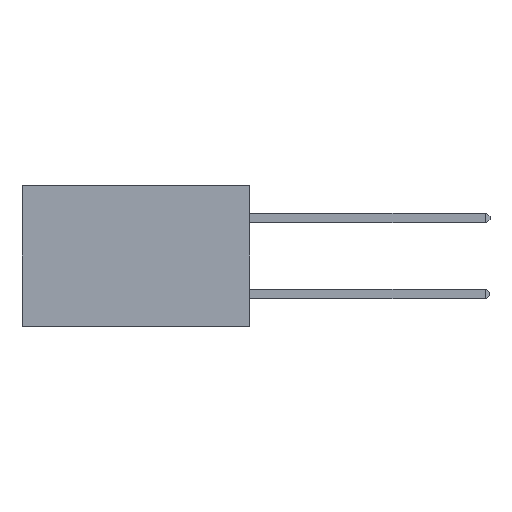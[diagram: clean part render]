
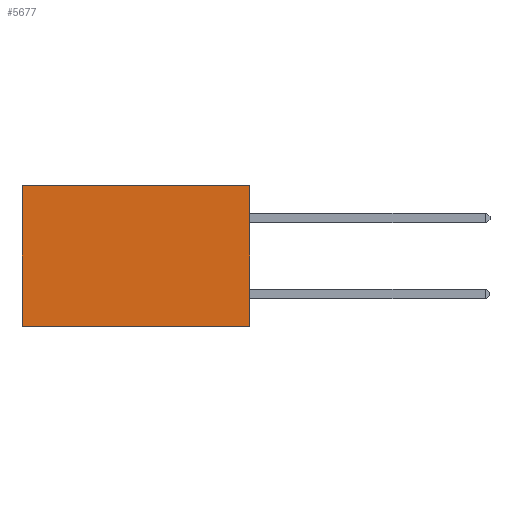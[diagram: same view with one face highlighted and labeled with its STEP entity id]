
A CAD part, left-side view. The second image highlights one B-rep face of the part: STEP entity #5677.
In plain terms, the highlighted planar face has unit normal (-1, 0, 0).
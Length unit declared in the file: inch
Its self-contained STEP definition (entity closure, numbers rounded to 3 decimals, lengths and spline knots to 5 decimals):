
#336 = CARTESIAN_POINT ( 'NONE',  ( 0.2875, 0.6, 0. ) ) ;
#605 = CARTESIAN_POINT ( 'NONE',  ( 0.2875, 0.6, 0. ) ) ;
#1169 = ORIENTED_EDGE ( 'NONE', *, *, #3508, .T. ) ;
#1212 = VECTOR ( 'NONE', #2059, 39.37008 ) ;
#2059 = DIRECTION ( 'NONE',  ( 0., 0., -1. ) ) ;
#2659 = FACE_OUTER_BOUND ( 'NONE', #3491, .T. ) ;
#2679 = CARTESIAN_POINT ( 'NONE',  ( 0.2875, 0., 0. ) ) ;
#2839 = ORIENTED_EDGE ( 'NONE', *, *, #12120, .T. ) ;
#3178 = EDGE_CURVE ( 'NONE', #4184, #4004, #9145, .T. ) ;
#3382 = DIRECTION ( 'NONE',  ( 0., 1., 0. ) ) ;
#3413 = CARTESIAN_POINT ( 'NONE',  ( 0.2875, 0., -0.37 ) ) ;
#3491 = EDGE_LOOP ( 'NONE', ( #2839, #12076, #4871, #1169 ) ) ;
#3508 = EDGE_CURVE ( 'NONE', #4184, #9931, #11908, .T. ) ;
#3695 = LINE ( 'NONE', #336, #11287 ) ;
#3715 = AXIS2_PLACEMENT_3D ( 'NONE', #2679, #11547, #5685 ) ;
#4004 = VERTEX_POINT ( 'NONE', #6241 ) ;
#4053 = VECTOR ( 'NONE', #10261, 39.37008 ) ;
#4184 = VERTEX_POINT ( 'NONE', #4662 ) ;
#4239 = EDGE_CURVE ( 'NONE', #4004, #8401, #5621, .T. ) ;
#4662 = CARTESIAN_POINT ( 'NONE',  ( 0.2875, 0., 0. ) ) ;
#4871 = ORIENTED_EDGE ( 'NONE', *, *, #3178, .F. ) ;
#5621 = LINE ( 'NONE', #3413, #8037 ) ;
#5677 = ADVANCED_FACE ( 'NONE', ( #2659 ), #6687, .F. ) ;
#5685 = DIRECTION ( 'NONE',  ( 0., 0., -1. ) ) ;
#6241 = CARTESIAN_POINT ( 'NONE',  ( 0.2875, 0., -0.37 ) ) ;
#6687 = PLANE ( 'NONE',  #3715 ) ;
#7156 = CARTESIAN_POINT ( 'NONE',  ( 0.2875, 0., 0. ) ) ;
#8037 = VECTOR ( 'NONE', #3382, 39.37008 ) ;
#8249 = DIRECTION ( 'NONE',  ( 0., 0., -1. ) ) ;
#8401 = VERTEX_POINT ( 'NONE', #11425 ) ;
#9145 = LINE ( 'NONE', #7156, #1212 ) ;
#9931 = VERTEX_POINT ( 'NONE', #605 ) ;
#10203 = CARTESIAN_POINT ( 'NONE',  ( 0.2875, 0., 0. ) ) ;
#10261 = DIRECTION ( 'NONE',  ( 0., 1., 0. ) ) ;
#11287 = VECTOR ( 'NONE', #8249, 39.37008 ) ;
#11425 = CARTESIAN_POINT ( 'NONE',  ( 0.2875, 0.6, -0.37 ) ) ;
#11547 = DIRECTION ( 'NONE',  ( 1., 0., 0. ) ) ;
#11908 = LINE ( 'NONE', #10203, #4053 ) ;
#12076 = ORIENTED_EDGE ( 'NONE', *, *, #4239, .F. ) ;
#12120 = EDGE_CURVE ( 'NONE', #9931, #8401, #3695, .T. ) ;
